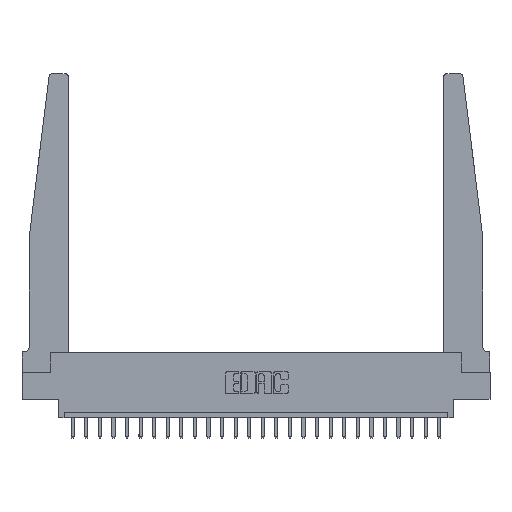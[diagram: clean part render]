
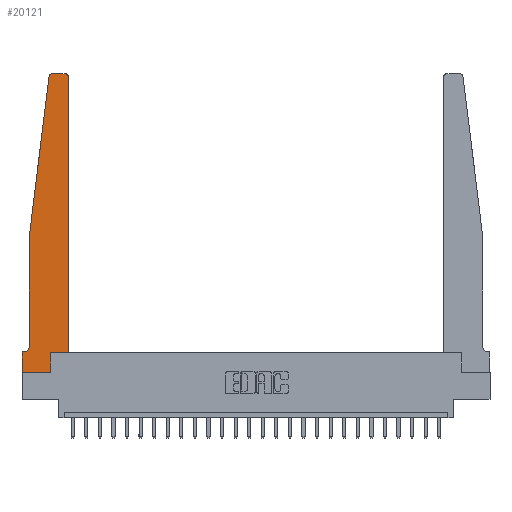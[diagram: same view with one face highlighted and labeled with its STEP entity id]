
A CAD part, top view. The second image highlights one B-rep face of the part: STEP entity #20121.
In plain terms, the highlighted planar face has unit normal (0, 0, 1).
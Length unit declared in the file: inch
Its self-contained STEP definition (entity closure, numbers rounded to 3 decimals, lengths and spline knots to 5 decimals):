
#79 = EDGE_CURVE ( 'NONE', #4022, #24556, #7769, .T. ) ;
#1321 = DIRECTION ( 'NONE',  ( 0., 0., 1. ) ) ;
#1672 = LINE ( 'NONE', #9294, #9033 ) ;
#1678 = DIRECTION ( 'NONE',  ( 1., 0., 0. ) ) ;
#1997 = DIRECTION ( 'NONE',  ( -1., 0., 0. ) ) ;
#2025 = ORIENTED_EDGE ( 'NONE', *, *, #9510, .T. ) ;
#2167 = DIRECTION ( 'NONE',  ( 0., 0., -1. ) ) ;
#2374 = ORIENTED_EDGE ( 'NONE', *, *, #10811, .T. ) ;
#2462 = DIRECTION ( 'NONE',  ( 1., 0., 0. ) ) ;
#2670 = VERTEX_POINT ( 'NONE', #20047 ) ;
#2702 = VECTOR ( 'NONE', #5075, 39.37008 ) ;
#3288 = ORIENTED_EDGE ( 'NONE', *, *, #7266, .T. ) ;
#3298 = DIRECTION ( 'NONE',  ( -0.122, -0.992, 0. ) ) ;
#3307 = PLANE ( 'NONE',  #19711 ) ;
#3591 = ORIENTED_EDGE ( 'NONE', *, *, #5929, .T. ) ;
#3627 = ORIENTED_EDGE ( 'NONE', *, *, #9782, .T. ) ;
#3657 = DIRECTION ( 'NONE',  ( 1., 0., 0. ) ) ;
#3753 = CARTESIAN_POINT ( 'NONE',  ( 0.425, 2.72, 0.37 ) ) ;
#3979 = LINE ( 'NONE', #16726, #4391 ) ;
#4022 = VERTEX_POINT ( 'NONE', #23683 ) ;
#4275 = ORIENTED_EDGE ( 'NONE', *, *, #15801, .T. ) ;
#4391 = VECTOR ( 'NONE', #11467, 39.37008 ) ;
#4592 = CARTESIAN_POINT ( 'NONE',  ( 0.425, 0.18, 0.37 ) ) ;
#5075 = DIRECTION ( 'NONE',  ( 0., -1., 0. ) ) ;
#5221 = VERTEX_POINT ( 'NONE', #19685 ) ;
#5224 = CARTESIAN_POINT ( 'NONE',  ( 0.015, 0.2375, 0.37 ) ) ;
#5466 = CIRCLE ( 'NONE', #9084, 0.05 ) ;
#5929 = EDGE_CURVE ( 'NONE', #2670, #5221, #11610, .T. ) ;
#6317 = DIRECTION ( 'NONE',  ( 0., 0., 1. ) ) ;
#6612 = ORIENTED_EDGE ( 'NONE', *, *, #9646, .T. ) ;
#6905 = CARTESIAN_POINT ( 'NONE',  ( 0., 0., 0.37 ) ) ;
#7186 = CARTESIAN_POINT ( 'NONE',  ( 0., 0., 0.37 ) ) ;
#7266 = EDGE_CURVE ( 'NONE', #24556, #2670, #12528, .T. ) ;
#7395 = CARTESIAN_POINT ( 'NONE',  ( 0.425, 0.18, 0.37 ) ) ;
#7492 = VERTEX_POINT ( 'NONE', #18000 ) ;
#7769 = LINE ( 'NONE', #7395, #10567 ) ;
#7897 = DIRECTION ( 'NONE',  ( 0., 1., 0. ) ) ;
#8073 = CARTESIAN_POINT ( 'NONE',  ( 0.27653, 2.72, 0.37 ) ) ;
#8771 = VERTEX_POINT ( 'NONE', #20637 ) ;
#9033 = VECTOR ( 'NONE', #19029, 39.37008 ) ;
#9084 = AXIS2_PLACEMENT_3D ( 'NONE', #5224, #2167, #9791 ) ;
#9294 = CARTESIAN_POINT ( 'NONE',  ( 0.2605, 0.18, 0.37 ) ) ;
#9411 = DIRECTION ( 'NONE',  ( 0., 0., 1. ) ) ;
#9432 = ORIENTED_EDGE ( 'NONE', *, *, #15714, .T. ) ;
#9510 = EDGE_CURVE ( 'NONE', #22927, #20092, #12080, .T. ) ;
#9646 = EDGE_CURVE ( 'NONE', #7492, #17235, #1672, .T. ) ;
#9782 = EDGE_CURVE ( 'NONE', #19512, #12412, #13892, .T. ) ;
#9791 = DIRECTION ( 'NONE',  ( -1., 0., 0. ) ) ;
#10567 = VECTOR ( 'NONE', #7897, 39.37008 ) ;
#10811 = EDGE_CURVE ( 'NONE', #21890, #8771, #5466, .T. ) ;
#11467 = DIRECTION ( 'NONE',  ( -1., 0., 0. ) ) ;
#11495 = ORIENTED_EDGE ( 'NONE', *, *, #18776, .T. ) ;
#11571 = VECTOR ( 'NONE', #2462, 39.37008 ) ;
#11610 = LINE ( 'NONE', #13115, #15424 ) ;
#12078 = LINE ( 'NONE', #4592, #11571 ) ;
#12080 = LINE ( 'NONE', #14535, #15002 ) ;
#12324 = LINE ( 'NONE', #16184, #2702 ) ;
#12412 = VERTEX_POINT ( 'NONE', #7186 ) ;
#12469 = AXIS2_PLACEMENT_3D ( 'NONE', #8073, #6317, #21567 ) ;
#12528 = CIRCLE ( 'NONE', #14908, 0.03 ) ;
#12554 = CARTESIAN_POINT ( 'NONE',  ( 0., 0.1875, 0.37 ) ) ;
#13115 = CARTESIAN_POINT ( 'NONE',  ( 0.25, 2.75, 0.37 ) ) ;
#13210 = ORIENTED_EDGE ( 'NONE', *, *, #13511, .T. ) ;
#13511 = EDGE_CURVE ( 'NONE', #20092, #21890, #12324, .T. ) ;
#13830 = CARTESIAN_POINT ( 'NONE',  ( 0., 0.1875, 0.37 ) ) ;
#13892 = LINE ( 'NONE', #23152, #22215 ) ;
#13976 = CARTESIAN_POINT ( 'NONE',  ( 0.065, 0.2375, 0.37 ) ) ;
#14516 = DIRECTION ( 'NONE',  ( 1., 0., 0. ) ) ;
#14535 = CARTESIAN_POINT ( 'NONE',  ( 0.065, 1.25, 0.37 ) ) ;
#14908 = AXIS2_PLACEMENT_3D ( 'NONE', #20780, #9411, #3657 ) ;
#14911 = VECTOR ( 'NONE', #14516, 39.37008 ) ;
#15002 = VECTOR ( 'NONE', #3298, 39.37008 ) ;
#15424 = VECTOR ( 'NONE', #1997, 39.37008 ) ;
#15624 = EDGE_LOOP ( 'NONE', ( #3591, #11495, #2025, #13210, #2374, #9432, #3627, #22315, #6612, #4275, #17646, #3288 ) ) ;
#15714 = EDGE_CURVE ( 'NONE', #8771, #19512, #3979, .T. ) ;
#15801 = EDGE_CURVE ( 'NONE', #17235, #4022, #12078, .T. ) ;
#16184 = CARTESIAN_POINT ( 'NONE',  ( 0.065, 1.25, 0.37 ) ) ;
#16504 = CARTESIAN_POINT ( 'NONE',  ( 0.24675, 2.72367, 0.37 ) ) ;
#16726 = CARTESIAN_POINT ( 'NONE',  ( 0.065, 0.1875, 0.37 ) ) ;
#17235 = VERTEX_POINT ( 'NONE', #23749 ) ;
#17646 = ORIENTED_EDGE ( 'NONE', *, *, #79, .T. ) ;
#18000 = CARTESIAN_POINT ( 'NONE',  ( 0.2605, 0., 0.37 ) ) ;
#18169 = CARTESIAN_POINT ( 'NONE',  ( 0.065, 1.25, 0.37 ) ) ;
#18776 = EDGE_CURVE ( 'NONE', #5221, #22927, #21664, .T. ) ;
#19029 = DIRECTION ( 'NONE',  ( 0., 1., 0. ) ) ;
#19512 = VERTEX_POINT ( 'NONE', #13830 ) ;
#19685 = CARTESIAN_POINT ( 'NONE',  ( 0.27653, 2.75, 0.37 ) ) ;
#19711 = AXIS2_PLACEMENT_3D ( 'NONE', #12554, #1321, #1678 ) ;
#20047 = CARTESIAN_POINT ( 'NONE',  ( 0.395, 2.75, 0.37 ) ) ;
#20092 = VERTEX_POINT ( 'NONE', #18169 ) ;
#20121 = ADVANCED_FACE ( 'NONE', ( #20320 ), #3307, .T. ) ;
#20320 = FACE_OUTER_BOUND ( 'NONE', #15624, .T. ) ;
#20637 = CARTESIAN_POINT ( 'NONE',  ( 0.015, 0.1875, 0.37 ) ) ;
#20682 = EDGE_CURVE ( 'NONE', #12412, #7492, #24035, .T. ) ;
#20780 = CARTESIAN_POINT ( 'NONE',  ( 0.395, 2.72, 0.37 ) ) ;
#21276 = DIRECTION ( 'NONE',  ( 0., -1., 0. ) ) ;
#21567 = DIRECTION ( 'NONE',  ( 1., 0., 0. ) ) ;
#21664 = CIRCLE ( 'NONE', #12469, 0.03 ) ;
#21890 = VERTEX_POINT ( 'NONE', #13976 ) ;
#22215 = VECTOR ( 'NONE', #21276, 39.37008 ) ;
#22315 = ORIENTED_EDGE ( 'NONE', *, *, #20682, .T. ) ;
#22927 = VERTEX_POINT ( 'NONE', #16504 ) ;
#23152 = CARTESIAN_POINT ( 'NONE',  ( 0., 0., 0.37 ) ) ;
#23683 = CARTESIAN_POINT ( 'NONE',  ( 0.425, 0.18, 0.37 ) ) ;
#23749 = CARTESIAN_POINT ( 'NONE',  ( 0.2605, 0.18, 0.37 ) ) ;
#24035 = LINE ( 'NONE', #6905, #14911 ) ;
#24556 = VERTEX_POINT ( 'NONE', #3753 ) ;
